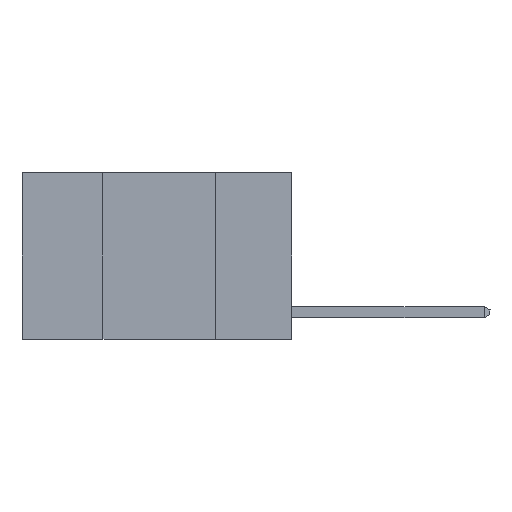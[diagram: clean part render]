
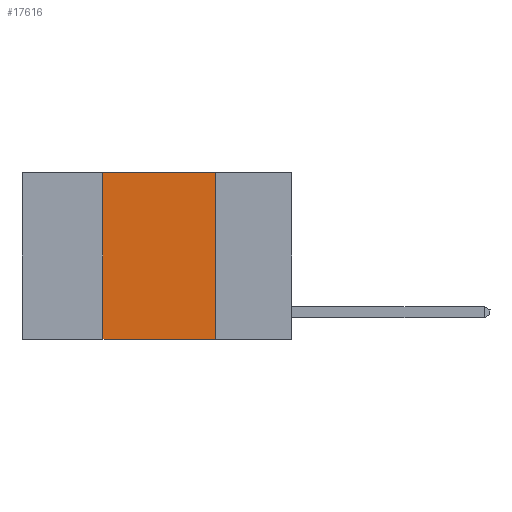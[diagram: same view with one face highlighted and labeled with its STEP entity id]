
A CAD part, left-side view. The second image highlights one B-rep face of the part: STEP entity #17616.
In plain terms, the highlighted planar face has unit normal (-1, 0, 0).
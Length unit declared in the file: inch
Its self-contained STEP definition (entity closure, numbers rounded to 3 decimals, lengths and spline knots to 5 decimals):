
#942 = CARTESIAN_POINT ( 'NONE',  ( 0., 0.17, 0. ) ) ;
#1152 = CARTESIAN_POINT ( 'NONE',  ( 0., 0.6, 0. ) ) ;
#3072 = ORIENTED_EDGE ( 'NONE', *, *, #6206, .F. ) ;
#3602 = CARTESIAN_POINT ( 'NONE',  ( 0., 0.42, 0. ) ) ;
#4408 = EDGE_LOOP ( 'NONE', ( #21600, #3072, #21603, #19327 ) ) ;
#5353 = EDGE_CURVE ( 'NONE', #11558, #8795, #24296, .T. ) ;
#6136 = DIRECTION ( 'NONE',  ( 0., 0., 1. ) ) ;
#6206 = EDGE_CURVE ( 'NONE', #8795, #20574, #24838, .T. ) ;
#6637 = EDGE_CURVE ( 'NONE', #20574, #10214, #24818, .T. ) ;
#7407 = CARTESIAN_POINT ( 'NONE',  ( 0., 0.17, 0. ) ) ;
#8795 = VERTEX_POINT ( 'NONE', #3602 ) ;
#8946 = PLANE ( 'NONE',  #16717 ) ;
#8969 = VECTOR ( 'NONE', #6136, 39.37008 ) ;
#10129 = VECTOR ( 'NONE', #22698, 39.37008 ) ;
#10214 = VERTEX_POINT ( 'NONE', #15356 ) ;
#10433 = FACE_OUTER_BOUND ( 'NONE', #4408, .T. ) ;
#11558 = VERTEX_POINT ( 'NONE', #12892 ) ;
#12578 = CARTESIAN_POINT ( 'NONE',  ( 0., 0.6, -0.37 ) ) ;
#12843 = DIRECTION ( 'NONE',  ( 0., 0., -1. ) ) ;
#12892 = CARTESIAN_POINT ( 'NONE',  ( 0., 0.42, -0.37 ) ) ;
#14595 = EDGE_CURVE ( 'NONE', #11558, #10214, #24690, .T. ) ;
#15356 = CARTESIAN_POINT ( 'NONE',  ( 0., 0.17, -0.37 ) ) ;
#15697 = DIRECTION ( 'NONE',  ( 0., -1., 0. ) ) ;
#15883 = VECTOR ( 'NONE', #15697, 39.37008 ) ;
#16717 = AXIS2_PLACEMENT_3D ( 'NONE', #1152, #24311, #12843 ) ;
#17616 = ADVANCED_FACE ( 'NONE', ( #10433 ), #8946, .F. ) ;
#18374 = DIRECTION ( 'NONE',  ( 0., -1., 0. ) ) ;
#19327 = ORIENTED_EDGE ( 'NONE', *, *, #14595, .T. ) ;
#19576 = CARTESIAN_POINT ( 'NONE',  ( 0., 0.42, 0. ) ) ;
#19608 = VECTOR ( 'NONE', #18374, 39.37008 ) ;
#20574 = VERTEX_POINT ( 'NONE', #942 ) ;
#21478 = CARTESIAN_POINT ( 'NONE',  ( 0., 0.6, 0. ) ) ;
#21600 = ORIENTED_EDGE ( 'NONE', *, *, #6637, .F. ) ;
#21603 = ORIENTED_EDGE ( 'NONE', *, *, #5353, .F. ) ;
#22698 = DIRECTION ( 'NONE',  ( 0., 0., -1. ) ) ;
#24296 = LINE ( 'NONE', #19576, #8969 ) ;
#24311 = DIRECTION ( 'NONE',  ( 1., 0., 0. ) ) ;
#24690 = LINE ( 'NONE', #12578, #19608 ) ;
#24818 = LINE ( 'NONE', #7407, #10129 ) ;
#24838 = LINE ( 'NONE', #21478, #15883 ) ;
